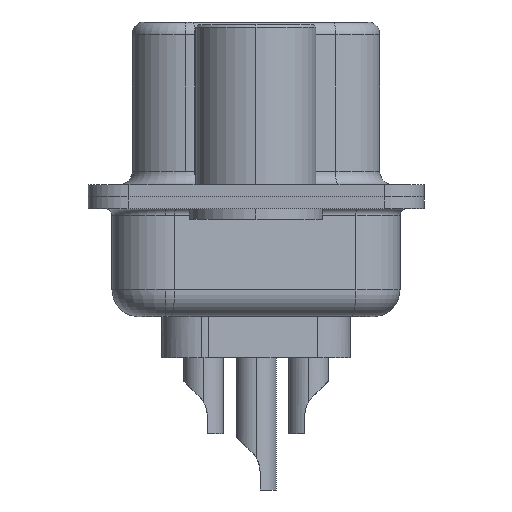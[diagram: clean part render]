
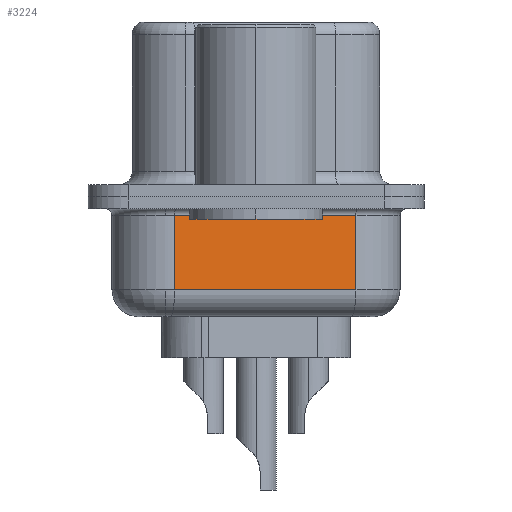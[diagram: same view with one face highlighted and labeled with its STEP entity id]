
A CAD part, left-side view. The second image highlights one B-rep face of the part: STEP entity #3224.
In plain terms, the highlighted planar face has unit normal (-0.985, -0.174, 0).
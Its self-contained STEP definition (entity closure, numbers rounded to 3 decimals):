
#127 = EDGE_CURVE ( 'NONE', #21610, #20520, #949, .T. ) ;
#786 = VECTOR ( 'NONE', #12079, 1000. ) ;
#949 = LINE ( 'NONE', #10516, #18674 ) ;
#3224 = ADVANCED_FACE ( 'NONE', ( #11837 ), #16383, .F. ) ;
#5819 = LINE ( 'NONE', #13733, #24051 ) ;
#6491 = CARTESIAN_POINT ( 'NONE',  ( 2.84, 3.053, -3.5 ) ) ;
#7119 = DIRECTION ( 'NONE',  ( -0.174, 0.985, 0. ) ) ;
#7182 = EDGE_LOOP ( 'NONE', ( #9116, #16630, #12904, #13708 ) ) ;
#8103 = LINE ( 'NONE', #6491, #786 ) ;
#9116 = ORIENTED_EDGE ( 'NONE', *, *, #24025, .F. ) ;
#9663 = DIRECTION ( 'NONE',  ( 0., 0., 1. ) ) ;
#10516 = CARTESIAN_POINT ( 'NONE',  ( 2.84, 3.053, -0.7 ) ) ;
#10839 = DIRECTION ( 'NONE',  ( 0.985, 0.174, 0. ) ) ;
#11099 = EDGE_CURVE ( 'NONE', #15181, #11638, #8103, .T. ) ;
#11638 = VERTEX_POINT ( 'NONE', #19659 ) ;
#11837 = FACE_OUTER_BOUND ( 'NONE', #7182, .T. ) ;
#12079 = DIRECTION ( 'NONE',  ( 0.174, -0.985, 0. ) ) ;
#12271 = LINE ( 'NONE', #22366, #18988 ) ;
#12379 = DIRECTION ( 'NONE',  ( -0.174, 0.985, 0. ) ) ;
#12904 = ORIENTED_EDGE ( 'NONE', *, *, #15165, .T. ) ;
#13708 = ORIENTED_EDGE ( 'NONE', *, *, #127, .T. ) ;
#13733 = CARTESIAN_POINT ( 'NONE',  ( 2.84, 3.053, -4.5 ) ) ;
#14490 = CARTESIAN_POINT ( 'NONE',  ( 2.84, 3.053, -3.5 ) ) ;
#14657 = CARTESIAN_POINT ( 'NONE',  ( 4.039, -3.747, -0.7 ) ) ;
#15165 = EDGE_CURVE ( 'NONE', #11638, #21610, #12271, .T. ) ;
#15181 = VERTEX_POINT ( 'NONE', #14490 ) ;
#16383 = PLANE ( 'NONE',  #20628 ) ;
#16630 = ORIENTED_EDGE ( 'NONE', *, *, #11099, .T. ) ;
#18170 = DIRECTION ( 'NONE',  ( 0., 0., 1. ) ) ;
#18674 = VECTOR ( 'NONE', #12379, 1000. ) ;
#18988 = VECTOR ( 'NONE', #18170, 1000. ) ;
#19659 = CARTESIAN_POINT ( 'NONE',  ( 4.039, -3.747, -3.5 ) ) ;
#20520 = VERTEX_POINT ( 'NONE', #23950 ) ;
#20628 = AXIS2_PLACEMENT_3D ( 'NONE', #23906, #10839, #7119 ) ;
#21610 = VERTEX_POINT ( 'NONE', #14657 ) ;
#22366 = CARTESIAN_POINT ( 'NONE',  ( 4.039, -3.747, -4.5 ) ) ;
#23906 = CARTESIAN_POINT ( 'NONE',  ( 2.84, 3.053, -4.5 ) ) ;
#23950 = CARTESIAN_POINT ( 'NONE',  ( 2.84, 3.053, -0.7 ) ) ;
#24025 = EDGE_CURVE ( 'NONE', #15181, #20520, #5819, .T. ) ;
#24051 = VECTOR ( 'NONE', #9663, 1000. ) ;
